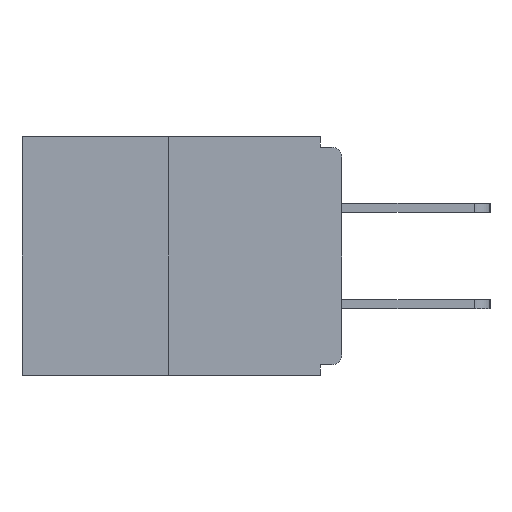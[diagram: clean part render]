
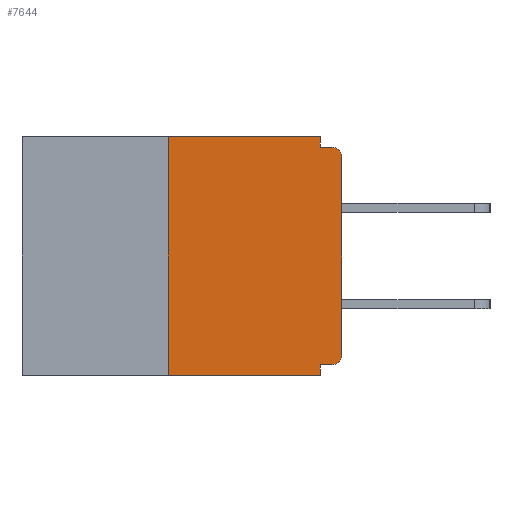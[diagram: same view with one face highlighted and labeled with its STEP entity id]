
A CAD part, left-side view. The second image highlights one B-rep face of the part: STEP entity #7644.
In plain terms, the highlighted planar face has unit normal (-1, 0, 0).
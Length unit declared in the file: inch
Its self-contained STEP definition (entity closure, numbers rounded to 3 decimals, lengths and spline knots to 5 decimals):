
#177 = DIRECTION ( 'NONE',  ( -1., 0., 0. ) ) ;
#271 = AXIS2_PLACEMENT_3D ( 'NONE', #23489, #21564, #3366 ) ;
#1039 = DIRECTION ( 'NONE',  ( 0., 0., 1. ) ) ;
#1117 = DIRECTION ( 'NONE',  ( 0., -1., 0. ) ) ;
#1156 = DIRECTION ( 'NONE',  ( 0., 0., -1. ) ) ;
#1449 = PLANE ( 'NONE',  #271 ) ;
#1518 = CARTESIAN_POINT ( 'NONE',  ( 0., 0., 0. ) ) ;
#2305 = CARTESIAN_POINT ( 'NONE',  ( 0., 0.031, -0.328 ) ) ;
#2442 = CARTESIAN_POINT ( 'NONE',  ( 0., 0.015, -0.313 ) ) ;
#2473 = VECTOR ( 'NONE', #7362, 39.37008 ) ;
#2542 = ORIENTED_EDGE ( 'NONE', *, *, #13205, .T. ) ;
#2904 = ORIENTED_EDGE ( 'NONE', *, *, #11670, .F. ) ;
#3366 = DIRECTION ( 'NONE',  ( 0., 0., -1. ) ) ;
#4014 = EDGE_CURVE ( 'NONE', #16142, #12361, #21164, .T. ) ;
#4054 = VECTOR ( 'NONE', #7335, 39.37008 ) ;
#4404 = CARTESIAN_POINT ( 'NONE',  ( 0., 0.015, -0.328 ) ) ;
#4601 = ORIENTED_EDGE ( 'NONE', *, *, #4014, .F. ) ;
#4694 = LINE ( 'NONE', #15996, #17990 ) ;
#5128 = ORIENTED_EDGE ( 'NONE', *, *, #6994, .T. ) ;
#5499 = DIRECTION ( 'NONE',  ( 0., 0., -1. ) ) ;
#5645 = ORIENTED_EDGE ( 'NONE', *, *, #7417, .T. ) ;
#5659 = VERTEX_POINT ( 'NONE', #12322 ) ;
#5822 = CARTESIAN_POINT ( 'NONE',  ( 0., 0.25, 0. ) ) ;
#5895 = DIRECTION ( 'NONE',  ( 0., 0., -1. ) ) ;
#6072 = VERTEX_POINT ( 'NONE', #10597 ) ;
#6159 = VERTEX_POINT ( 'NONE', #18270 ) ;
#6994 = EDGE_CURVE ( 'NONE', #23276, #6159, #22854, .T. ) ;
#7076 = ORIENTED_EDGE ( 'NONE', *, *, #10647, .F. ) ;
#7335 = DIRECTION ( 'NONE',  ( 0., -1., 0. ) ) ;
#7362 = DIRECTION ( 'NONE',  ( 0., -1., 0. ) ) ;
#7417 = EDGE_CURVE ( 'NONE', #16142, #6072, #11301, .T. ) ;
#7600 = DIRECTION ( 'NONE',  ( 0., 0., 1. ) ) ;
#7644 = ADVANCED_FACE ( 'NONE', ( #14310 ), #1449, .F. ) ;
#8563 = VECTOR ( 'NONE', #16067, 39.37008 ) ;
#8718 = CARTESIAN_POINT ( 'NONE',  ( 0., 0.031, -0.343 ) ) ;
#9429 = VERTEX_POINT ( 'NONE', #23677 ) ;
#9810 = ORIENTED_EDGE ( 'NONE', *, *, #21515, .F. ) ;
#10197 = AXIS2_PLACEMENT_3D ( 'NONE', #14705, #177, #11216 ) ;
#10597 = CARTESIAN_POINT ( 'NONE',  ( 0., 0.031, -0.343 ) ) ;
#10647 = EDGE_CURVE ( 'NONE', #20183, #6072, #23085, .T. ) ;
#11057 = ORIENTED_EDGE ( 'NONE', *, *, #22204, .F. ) ;
#11216 = DIRECTION ( 'NONE',  ( 0., 0., -1. ) ) ;
#11292 = CARTESIAN_POINT ( 'NONE',  ( 0., 0.015, -0.015 ) ) ;
#11301 = LINE ( 'NONE', #11433, #4054 ) ;
#11433 = CARTESIAN_POINT ( 'NONE',  ( 0., 0.46, -0.343 ) ) ;
#11670 = EDGE_CURVE ( 'NONE', #5659, #22417, #19801, .T. ) ;
#11872 = CARTESIAN_POINT ( 'NONE',  ( 0., 0.25, -0.343 ) ) ;
#12322 = CARTESIAN_POINT ( 'NONE',  ( 0., 0.031, 0. ) ) ;
#12361 = VERTEX_POINT ( 'NONE', #5822 ) ;
#12551 = AXIS2_PLACEMENT_3D ( 'NONE', #2442, #17097, #5895 ) ;
#12917 = LINE ( 'NONE', #16509, #2473 ) ;
#12967 = VECTOR ( 'NONE', #1039, 39.37008 ) ;
#12981 = VECTOR ( 'NONE', #7600, 39.37008 ) ;
#13205 = EDGE_CURVE ( 'NONE', #6159, #9429, #18426, .T. ) ;
#13303 = VECTOR ( 'NONE', #5499, 39.37008 ) ;
#13715 = ORIENTED_EDGE ( 'NONE', *, *, #15202, .F. ) ;
#14310 = FACE_OUTER_BOUND ( 'NONE', #21669, .T. ) ;
#14658 = CARTESIAN_POINT ( 'NONE',  ( 0., 0.031, 0. ) ) ;
#14678 = VERTEX_POINT ( 'NONE', #11292 ) ;
#14705 = CARTESIAN_POINT ( 'NONE',  ( 0., 0.015, -0.03 ) ) ;
#14797 = VECTOR ( 'NONE', #1156, 39.37008 ) ;
#15202 = EDGE_CURVE ( 'NONE', #22417, #14678, #4694, .T. ) ;
#15996 = CARTESIAN_POINT ( 'NONE',  ( 0., 0., -0.015 ) ) ;
#16067 = DIRECTION ( 'NONE',  ( 0., 1., 0. ) ) ;
#16142 = VERTEX_POINT ( 'NONE', #11872 ) ;
#16509 = CARTESIAN_POINT ( 'NONE',  ( 0., 0.46, 0. ) ) ;
#17097 = DIRECTION ( 'NONE',  ( -1., 0., 0. ) ) ;
#17631 = CARTESIAN_POINT ( 'NONE',  ( 0., 0.25, 0. ) ) ;
#17990 = VECTOR ( 'NONE', #1117, 39.37008 ) ;
#18102 = ORIENTED_EDGE ( 'NONE', *, *, #22849, .T. ) ;
#18270 = CARTESIAN_POINT ( 'NONE',  ( 0., 0., -0.313 ) ) ;
#18343 = CARTESIAN_POINT ( 'NONE',  ( 0., 0.031, -0.015 ) ) ;
#18426 = LINE ( 'NONE', #1518, #12981 ) ;
#19535 = CARTESIAN_POINT ( 'NONE',  ( 0., 0., -0.328 ) ) ;
#19801 = LINE ( 'NONE', #14658, #13303 ) ;
#20183 = VERTEX_POINT ( 'NONE', #2305 ) ;
#20898 = CIRCLE ( 'NONE', #10197, 0.015 ) ;
#21164 = LINE ( 'NONE', #17631, #12967 ) ;
#21195 = LINE ( 'NONE', #19535, #8563 ) ;
#21515 = EDGE_CURVE ( 'NONE', #12361, #5659, #12917, .T. ) ;
#21564 = DIRECTION ( 'NONE',  ( 1., 0., 0. ) ) ;
#21669 = EDGE_LOOP ( 'NONE', ( #9810, #4601, #5645, #7076, #11057, #5128, #2542, #18102, #13715, #2904 ) ) ;
#22204 = EDGE_CURVE ( 'NONE', #23276, #20183, #21195, .T. ) ;
#22417 = VERTEX_POINT ( 'NONE', #18343 ) ;
#22849 = EDGE_CURVE ( 'NONE', #9429, #14678, #20898, .T. ) ;
#22854 = CIRCLE ( 'NONE', #12551, 0.015 ) ;
#23085 = LINE ( 'NONE', #8718, #14797 ) ;
#23276 = VERTEX_POINT ( 'NONE', #4404 ) ;
#23489 = CARTESIAN_POINT ( 'NONE',  ( 0., 0.46, 0. ) ) ;
#23677 = CARTESIAN_POINT ( 'NONE',  ( 0., 0., -0.03 ) ) ;
